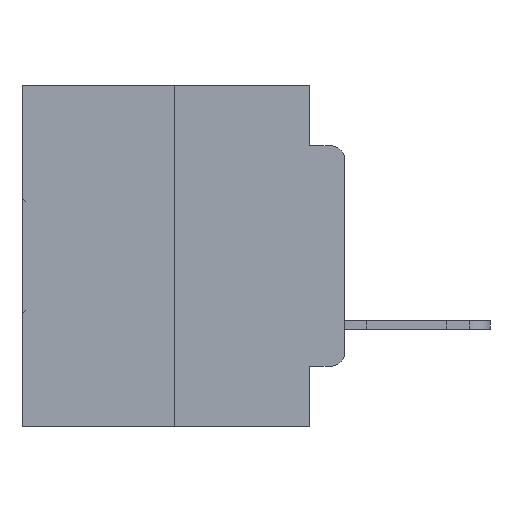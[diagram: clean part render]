
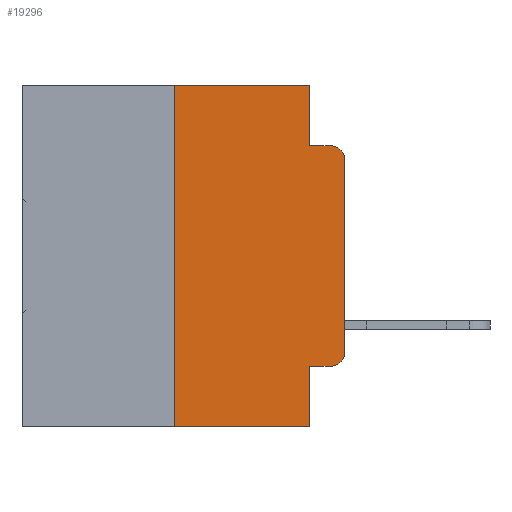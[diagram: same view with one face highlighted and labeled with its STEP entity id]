
A CAD part, left-side view. The second image highlights one B-rep face of the part: STEP entity #19296.
In plain terms, the highlighted planar face has unit normal (-1, 0, 0).
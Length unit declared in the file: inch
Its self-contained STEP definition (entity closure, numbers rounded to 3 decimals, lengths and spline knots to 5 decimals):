
#646 = CARTESIAN_POINT ( 'NONE',  ( 0., 0.473, 0. ) ) ;
#667 = CARTESIAN_POINT ( 'NONE',  ( 0., 0.051, -0.5 ) ) ;
#737 = DIRECTION ( 'NONE',  ( 0., -1., 0. ) ) ;
#1508 = VERTEX_POINT ( 'NONE', #11249 ) ;
#1636 = EDGE_CURVE ( 'NONE', #23954, #1508, #28244, .T. ) ;
#2104 = DIRECTION ( 'NONE',  ( 0., 0., -1. ) ) ;
#2653 = VECTOR ( 'NONE', #19135, 39.37008 ) ;
#2729 = AXIS2_PLACEMENT_3D ( 'NONE', #17739, #5723, #5387 ) ;
#3041 = PLANE ( 'NONE',  #24509 ) ;
#3320 = VECTOR ( 'NONE', #737, 39.37008 ) ;
#3739 = CARTESIAN_POINT ( 'NONE',  ( 0., 0.25, 0. ) ) ;
#3763 = ORIENTED_EDGE ( 'NONE', *, *, #19712, .T. ) ;
#3993 = VERTEX_POINT ( 'NONE', #24495 ) ;
#4044 = ORIENTED_EDGE ( 'NONE', *, *, #23401, .F. ) ;
#4084 = LINE ( 'NONE', #8458, #3320 ) ;
#4668 = EDGE_CURVE ( 'NONE', #18874, #11939, #19596, .T. ) ;
#4683 = VERTEX_POINT ( 'NONE', #17518 ) ;
#4856 = AXIS2_PLACEMENT_3D ( 'NONE', #30349, #9793, #2104 ) ;
#5387 = DIRECTION ( 'NONE',  ( 0., 0., -1. ) ) ;
#5723 = DIRECTION ( 'NONE',  ( -1., 0., 0. ) ) ;
#7262 = DIRECTION ( 'NONE',  ( 0., -1., 0. ) ) ;
#7572 = DIRECTION ( 'NONE',  ( 0., -1., 0. ) ) ;
#7874 = CARTESIAN_POINT ( 'NONE',  ( 0., 0., -0.1085 ) ) ;
#8458 = CARTESIAN_POINT ( 'NONE',  ( 0., 0.051, -0.0885 ) ) ;
#9286 = LINE ( 'NONE', #9424, #25959 ) ;
#9424 = CARTESIAN_POINT ( 'NONE',  ( 0., 0.473, -0.5 ) ) ;
#9793 = DIRECTION ( 'NONE',  ( -1., 0., 0. ) ) ;
#10196 = ORIENTED_EDGE ( 'NONE', *, *, #31917, .T. ) ;
#10587 = CARTESIAN_POINT ( 'NONE',  ( 0., 0.25, 0. ) ) ;
#10697 = CARTESIAN_POINT ( 'NONE',  ( 0., 0.051, 0. ) ) ;
#11249 = CARTESIAN_POINT ( 'NONE',  ( 0., 0., -0.3915 ) ) ;
#11360 = ORIENTED_EDGE ( 'NONE', *, *, #17676, .F. ) ;
#11435 = CARTESIAN_POINT ( 'NONE',  ( 0., 0., 0. ) ) ;
#11939 = VERTEX_POINT ( 'NONE', #21516 ) ;
#12555 = ORIENTED_EDGE ( 'NONE', *, *, #4668, .F. ) ;
#12865 = VECTOR ( 'NONE', #27895, 39.37008 ) ;
#14112 = VERTEX_POINT ( 'NONE', #667 ) ;
#14247 = ORIENTED_EDGE ( 'NONE', *, *, #1636, .T. ) ;
#15607 = LINE ( 'NONE', #25518, #20683 ) ;
#16545 = EDGE_CURVE ( 'NONE', #4683, #14112, #17603, .T. ) ;
#16629 = CARTESIAN_POINT ( 'NONE',  ( 0., 0.051, -0.4115 ) ) ;
#17518 = CARTESIAN_POINT ( 'NONE',  ( 0., 0.051, -0.4115 ) ) ;
#17603 = LINE ( 'NONE', #10697, #29225 ) ;
#17676 = EDGE_CURVE ( 'NONE', #11939, #3993, #15607, .T. ) ;
#17739 = CARTESIAN_POINT ( 'NONE',  ( 0., 0.02, -0.1085 ) ) ;
#17826 = EDGE_CURVE ( 'NONE', #25475, #18874, #31124, .T. ) ;
#18110 = DIRECTION ( 'NONE',  ( 0., 0., -1. ) ) ;
#18635 = LINE ( 'NONE', #11435, #20215 ) ;
#18874 = VERTEX_POINT ( 'NONE', #3739 ) ;
#19016 = DIRECTION ( 'NONE',  ( 0., 0., 1. ) ) ;
#19036 = ORIENTED_EDGE ( 'NONE', *, *, #31640, .T. ) ;
#19135 = DIRECTION ( 'NONE',  ( 0., -1., 0. ) ) ;
#19296 = ADVANCED_FACE ( 'NONE', ( #29454 ), #3041, .F. ) ;
#19596 = LINE ( 'NONE', #29959, #21159 ) ;
#19712 = EDGE_CURVE ( 'NONE', #25475, #14112, #9286, .T. ) ;
#20125 = CARTESIAN_POINT ( 'NONE',  ( 0., 0.02, -0.0885 ) ) ;
#20215 = VECTOR ( 'NONE', #19016, 39.37008 ) ;
#20683 = VECTOR ( 'NONE', #27978, 39.37008 ) ;
#21159 = VECTOR ( 'NONE', #7572, 39.37008 ) ;
#21516 = CARTESIAN_POINT ( 'NONE',  ( 0., 0.051, 0. ) ) ;
#22672 = DIRECTION ( 'NONE',  ( 1., 0., 0. ) ) ;
#23401 = EDGE_CURVE ( 'NONE', #3993, #28674, #4084, .T. ) ;
#23954 = VERTEX_POINT ( 'NONE', #28019 ) ;
#24495 = CARTESIAN_POINT ( 'NONE',  ( 0., 0.051, -0.0885 ) ) ;
#24509 = AXIS2_PLACEMENT_3D ( 'NONE', #646, #22672, #18110 ) ;
#24851 = ORIENTED_EDGE ( 'NONE', *, *, #17826, .F. ) ;
#25031 = VERTEX_POINT ( 'NONE', #7874 ) ;
#25376 = ORIENTED_EDGE ( 'NONE', *, *, #30182, .T. ) ;
#25426 = DIRECTION ( 'NONE',  ( 0., 0., -1. ) ) ;
#25475 = VERTEX_POINT ( 'NONE', #26588 ) ;
#25518 = CARTESIAN_POINT ( 'NONE',  ( 0., 0.051, 0. ) ) ;
#25959 = VECTOR ( 'NONE', #7262, 39.37008 ) ;
#26053 = EDGE_LOOP ( 'NONE', ( #25376, #19036, #4044, #11360, #12555, #24851, #3763, #28668, #10196, #14247 ) ) ;
#26588 = CARTESIAN_POINT ( 'NONE',  ( 0., 0.25, -0.5 ) ) ;
#26727 = CIRCLE ( 'NONE', #2729, 0.02 ) ;
#27895 = DIRECTION ( 'NONE',  ( 0., 0., 1. ) ) ;
#27978 = DIRECTION ( 'NONE',  ( 0., 0., -1. ) ) ;
#28019 = CARTESIAN_POINT ( 'NONE',  ( 0., 0.02, -0.4115 ) ) ;
#28244 = CIRCLE ( 'NONE', #4856, 0.02 ) ;
#28668 = ORIENTED_EDGE ( 'NONE', *, *, #16545, .F. ) ;
#28674 = VERTEX_POINT ( 'NONE', #20125 ) ;
#29225 = VECTOR ( 'NONE', #25426, 39.37008 ) ;
#29454 = FACE_OUTER_BOUND ( 'NONE', #26053, .T. ) ;
#29959 = CARTESIAN_POINT ( 'NONE',  ( 0., 0.473, 0. ) ) ;
#30182 = EDGE_CURVE ( 'NONE', #1508, #25031, #18635, .T. ) ;
#30349 = CARTESIAN_POINT ( 'NONE',  ( 0., 0.02, -0.3915 ) ) ;
#30575 = LINE ( 'NONE', #16629, #2653 ) ;
#31124 = LINE ( 'NONE', #10587, #12865 ) ;
#31640 = EDGE_CURVE ( 'NONE', #25031, #28674, #26727, .T. ) ;
#31917 = EDGE_CURVE ( 'NONE', #4683, #23954, #30575, .T. ) ;
